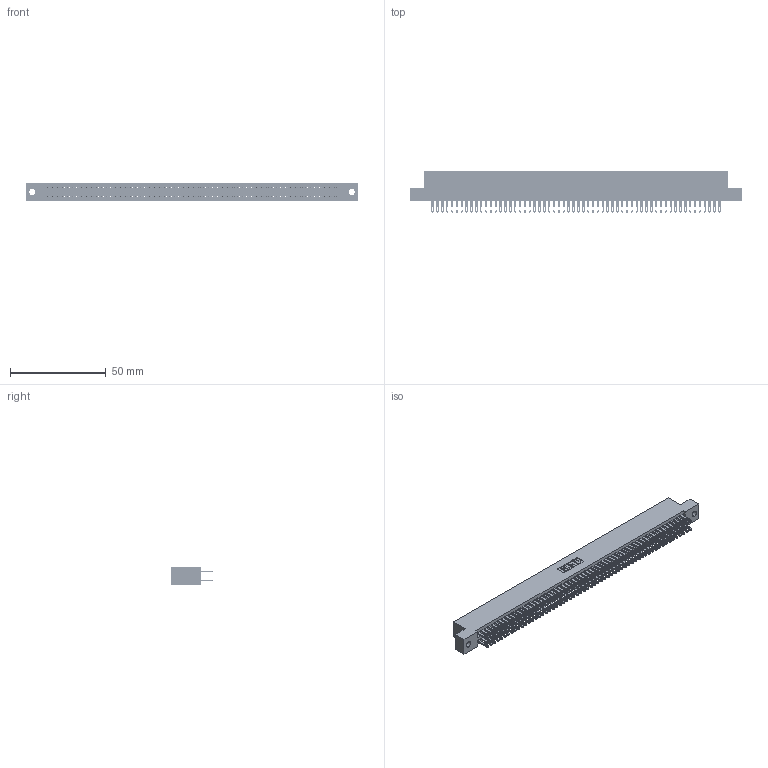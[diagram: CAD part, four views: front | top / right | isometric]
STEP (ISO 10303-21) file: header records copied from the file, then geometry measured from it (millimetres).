
FILE_DESCRIPTION (( 'STEP AP203' ), '1' );
FILE_NAME ('845-120-500-202.STEP', '2018-11-21T00:28:17', ( '' ), ( '' ), 'SwSTEP 2.0', 'SolidWorks 2016', '' );
FILE_SCHEMA (( 'CONFIG_CONTROL_DESIGN' ));
Length unit declared in the file: inch
Products named in the file (3): 845 Part_Flush Mounting Lugs - 0.128 Dia; 345-292-001_345-293-100; 845-120-500-202
Assembly tree (121 placements, depth 2):
  845-120-500-202
    845 Part_Flush Mounting Lugs - 0.128 Dia
    345-292-001_345-293-100  x120
Bounding box: 173.61 x 21.51 x 9.4 mm (x, y, z)
Volume: 17361.7 mm3; surface area: 26963.3 mm2
Topology: 121 solids, 121 shells, 5646 faces, 17261 edges, 11506 vertices
Faces by surface type: plane 3320, cylinder 2326
Entity records: 44587 total; most frequent: CARTESIAN_POINT 7456, ORIENTED_EDGE 7390, DIRECTION 6555, EDGE_CURVE 3695, VECTOR 3319, LINE 3319, VERTEX_POINT 2462, AXIS2_PLACEMENT_3D 1618
